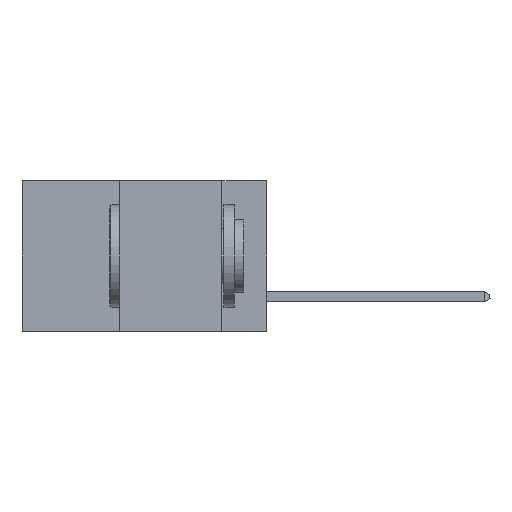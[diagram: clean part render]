
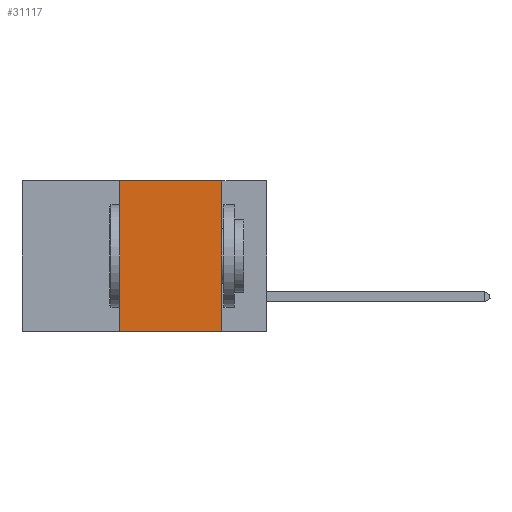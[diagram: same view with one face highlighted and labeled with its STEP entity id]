
A CAD part, left-side view. The second image highlights one B-rep face of the part: STEP entity #31117.
In plain terms, the highlighted planar face has unit normal (-1, 0, 0).
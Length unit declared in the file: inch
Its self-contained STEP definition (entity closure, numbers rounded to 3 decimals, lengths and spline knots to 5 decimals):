
#3360 = CARTESIAN_POINT ( 'NONE',  ( 0., 0.36, -0.37 ) ) ;
#3421 = CARTESIAN_POINT ( 'NONE',  ( 0., 0.11, -0.37 ) ) ;
#4949 = LINE ( 'NONE', #38271, #23068 ) ;
#8950 = CARTESIAN_POINT ( 'NONE',  ( 0., 0.6, 0. ) ) ;
#10307 = ORIENTED_EDGE ( 'NONE', *, *, #26457, .F. ) ;
#11711 = DIRECTION ( 'NONE',  ( 0., 0., -1. ) ) ;
#12097 = CARTESIAN_POINT ( 'NONE',  ( 0., 0.6, 0. ) ) ;
#15240 = VERTEX_POINT ( 'NONE', #16996 ) ;
#15247 = VECTOR ( 'NONE', #31368, 39.37008 ) ;
#15298 = CARTESIAN_POINT ( 'NONE',  ( 0., 0.36, 0. ) ) ;
#15396 = VERTEX_POINT ( 'NONE', #15298 ) ;
#16573 = EDGE_CURVE ( 'NONE', #37304, #32531, #4949, .T. ) ;
#16996 = CARTESIAN_POINT ( 'NONE',  ( 0., 0.11, 0. ) ) ;
#17644 = PLANE ( 'NONE',  #20821 ) ;
#18655 = LINE ( 'NONE', #12097, #30297 ) ;
#20821 = AXIS2_PLACEMENT_3D ( 'NONE', #8950, #35250, #11711 ) ;
#22162 = CARTESIAN_POINT ( 'NONE',  ( 0., 0.11, 0. ) ) ;
#22288 = DIRECTION ( 'NONE',  ( 0., 0., -1. ) ) ;
#23068 = VECTOR ( 'NONE', #31737, 39.37008 ) ;
#23147 = LINE ( 'NONE', #34376, #15247 ) ;
#23451 = EDGE_LOOP ( 'NONE', ( #31207, #10307, #24285, #30437 ) ) ;
#24285 = ORIENTED_EDGE ( 'NONE', *, *, #38084, .F. ) ;
#26457 = EDGE_CURVE ( 'NONE', #15396, #15240, #18655, .T. ) ;
#26582 = LINE ( 'NONE', #22162, #31712 ) ;
#30297 = VECTOR ( 'NONE', #36285, 39.37008 ) ;
#30437 = ORIENTED_EDGE ( 'NONE', *, *, #16573, .T. ) ;
#31026 = FACE_OUTER_BOUND ( 'NONE', #23451, .T. ) ;
#31117 = ADVANCED_FACE ( 'NONE', ( #31026 ), #17644, .F. ) ;
#31207 = ORIENTED_EDGE ( 'NONE', *, *, #35690, .F. ) ;
#31368 = DIRECTION ( 'NONE',  ( 0., 0., 1. ) ) ;
#31712 = VECTOR ( 'NONE', #22288, 39.37008 ) ;
#31737 = DIRECTION ( 'NONE',  ( 0., -1., 0. ) ) ;
#32531 = VERTEX_POINT ( 'NONE', #3421 ) ;
#34376 = CARTESIAN_POINT ( 'NONE',  ( 0., 0.36, 0. ) ) ;
#35250 = DIRECTION ( 'NONE',  ( 1., 0., 0. ) ) ;
#35690 = EDGE_CURVE ( 'NONE', #15240, #32531, #26582, .T. ) ;
#36285 = DIRECTION ( 'NONE',  ( 0., -1., 0. ) ) ;
#37304 = VERTEX_POINT ( 'NONE', #3360 ) ;
#38084 = EDGE_CURVE ( 'NONE', #37304, #15396, #23147, .T. ) ;
#38271 = CARTESIAN_POINT ( 'NONE',  ( 0., 0.6, -0.37 ) ) ;
